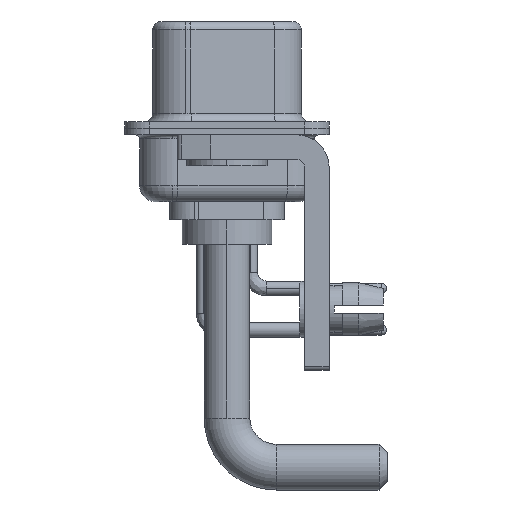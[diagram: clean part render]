
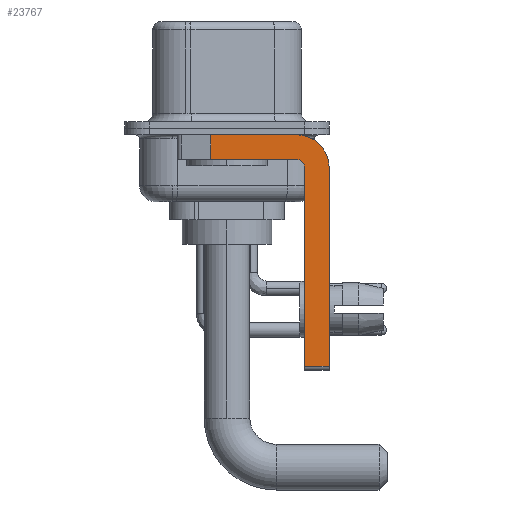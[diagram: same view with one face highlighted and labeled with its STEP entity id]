
A CAD part, left-side view. The second image highlights one B-rep face of the part: STEP entity #23767.
In plain terms, the highlighted planar face has unit normal (-1, 0, 0).
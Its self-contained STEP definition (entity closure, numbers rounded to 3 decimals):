
#248 = VERTEX_POINT ( 'NONE', #5259 ) ;
#387 = VERTEX_POINT ( 'NONE', #3682 ) ;
#442 = CARTESIAN_POINT ( 'NONE',  ( -2.9, -4.25, -2.4 ) ) ;
#1181 = ORIENTED_EDGE ( 'NONE', *, *, #1899, .F. ) ;
#1442 = VECTOR ( 'NONE', #6061, 1000. ) ;
#1899 = EDGE_CURVE ( 'NONE', #14239, #23284, #9197, .T. ) ;
#1978 = CARTESIAN_POINT ( 'NONE',  ( -2.9, -4.25, -1.9 ) ) ;
#2031 = ORIENTED_EDGE ( 'NONE', *, *, #20994, .T. ) ;
#2610 = DIRECTION ( 'NONE',  ( 1., 0., 0. ) ) ;
#2784 = VECTOR ( 'NONE', #12528, 1000. ) ;
#2988 = VERTEX_POINT ( 'NONE', #27002 ) ;
#3682 = CARTESIAN_POINT ( 'NONE',  ( -2.9, -4.75, -14.55 ) ) ;
#3792 = CIRCLE ( 'NONE', #19423, 0.5 ) ;
#3878 = CARTESIAN_POINT ( 'NONE',  ( -2.9, 0.978, -1.9 ) ) ;
#4017 = CARTESIAN_POINT ( 'NONE',  ( -2.9, 3., -0.4 ) ) ;
#4166 = CARTESIAN_POINT ( 'NONE',  ( -2.9, -4.25, -1.9 ) ) ;
#4299 = CARTESIAN_POINT ( 'NONE',  ( -2.9, -4.25, -2.4 ) ) ;
#4890 = CARTESIAN_POINT ( 'NONE',  ( -2.9, 0.978, -1.9 ) ) ;
#5004 = DIRECTION ( 'NONE',  ( 0., 1., 0. ) ) ;
#5259 = CARTESIAN_POINT ( 'NONE',  ( -2.9, -4.25, -0.4 ) ) ;
#6061 = DIRECTION ( 'NONE',  ( 0., -1., 0. ) ) ;
#6113 = VERTEX_POINT ( 'NONE', #12465 ) ;
#6408 = DIRECTION ( 'NONE',  ( 0., 0., -1. ) ) ;
#7943 = EDGE_LOOP ( 'NONE', ( #17650, #2031, #21225, #16531, #19370, #17095, #1181, #20804 ) ) ;
#9197 = LINE ( 'NONE', #11328, #11193 ) ;
#9344 = DIRECTION ( 'NONE',  ( 0., 0., 1. ) ) ;
#11096 = EDGE_CURVE ( 'NONE', #6113, #14680, #3792, .T. ) ;
#11193 = VECTOR ( 'NONE', #26929, 1000. ) ;
#11247 = DIRECTION ( 'NONE',  ( 1., 0., 0. ) ) ;
#11328 = CARTESIAN_POINT ( 'NONE',  ( -2.9, -6.25, -2.4 ) ) ;
#12465 = CARTESIAN_POINT ( 'NONE',  ( -2.9, -4.75, -2.4 ) ) ;
#12528 = DIRECTION ( 'NONE',  ( 0., -1., 0. ) ) ;
#12586 = LINE ( 'NONE', #18972, #1442 ) ;
#13362 = EDGE_CURVE ( 'NONE', #2988, #248, #25722, .T. ) ;
#14239 = VERTEX_POINT ( 'NONE', #25405 ) ;
#14680 = VERTEX_POINT ( 'NONE', #1978 ) ;
#14869 = AXIS2_PLACEMENT_3D ( 'NONE', #4299, #2610, #6408 ) ;
#15416 = CARTESIAN_POINT ( 'NONE',  ( -2.9, -4.75, -14.8 ) ) ;
#15484 = EDGE_CURVE ( 'NONE', #387, #23284, #12586, .T. ) ;
#15589 = DIRECTION ( 'NONE',  ( -1., 0., 0. ) ) ;
#16090 = VERTEX_POINT ( 'NONE', #3878 ) ;
#16531 = ORIENTED_EDGE ( 'NONE', *, *, #11096, .F. ) ;
#17095 = ORIENTED_EDGE ( 'NONE', *, *, #15484, .T. ) ;
#17592 = CIRCLE ( 'NONE', #14869, 2. ) ;
#17650 = ORIENTED_EDGE ( 'NONE', *, *, #13362, .F. ) ;
#17831 = LINE ( 'NONE', #15416, #20067 ) ;
#18037 = DIRECTION ( 'NONE',  ( 0., 0., -1. ) ) ;
#18972 = CARTESIAN_POINT ( 'NONE',  ( -2.9, -4.25, -14.55 ) ) ;
#19370 = ORIENTED_EDGE ( 'NONE', *, *, #26095, .F. ) ;
#19423 = AXIS2_PLACEMENT_3D ( 'NONE', #442, #15589, #9344 ) ;
#19554 = VECTOR ( 'NONE', #5004, 1000. ) ;
#20067 = VECTOR ( 'NONE', #24085, 1000. ) ;
#20804 = ORIENTED_EDGE ( 'NONE', *, *, #22582, .F. ) ;
#20908 = AXIS2_PLACEMENT_3D ( 'NONE', #22163, #11247, #18037 ) ;
#20994 = EDGE_CURVE ( 'NONE', #2988, #16090, #24322, .T. ) ;
#21075 = VECTOR ( 'NONE', #22179, 1000. ) ;
#21225 = ORIENTED_EDGE ( 'NONE', *, *, #23686, .F. ) ;
#22163 = CARTESIAN_POINT ( 'NONE',  ( -2.9, -4.25, -2.4 ) ) ;
#22179 = DIRECTION ( 'NONE',  ( 0., 0., -1. ) ) ;
#22305 = PLANE ( 'NONE',  #20908 ) ;
#22582 = EDGE_CURVE ( 'NONE', #248, #14239, #17592, .T. ) ;
#22751 = CARTESIAN_POINT ( 'NONE',  ( -2.9, -6.25, -14.55 ) ) ;
#23284 = VERTEX_POINT ( 'NONE', #22751 ) ;
#23582 = LINE ( 'NONE', #4166, #19554 ) ;
#23686 = EDGE_CURVE ( 'NONE', #14680, #16090, #23582, .T. ) ;
#23767 = ADVANCED_FACE ( 'NONE', ( #24436 ), #22305, .F. ) ;
#24085 = DIRECTION ( 'NONE',  ( 0., 0., 1. ) ) ;
#24322 = LINE ( 'NONE', #4890, #21075 ) ;
#24436 = FACE_OUTER_BOUND ( 'NONE', #7943, .T. ) ;
#25405 = CARTESIAN_POINT ( 'NONE',  ( -2.9, -6.25, -2.4 ) ) ;
#25722 = LINE ( 'NONE', #4017, #2784 ) ;
#26095 = EDGE_CURVE ( 'NONE', #387, #6113, #17831, .T. ) ;
#26929 = DIRECTION ( 'NONE',  ( 0., 0., -1. ) ) ;
#27002 = CARTESIAN_POINT ( 'NONE',  ( -2.9, 0.978, -0.4 ) ) ;
